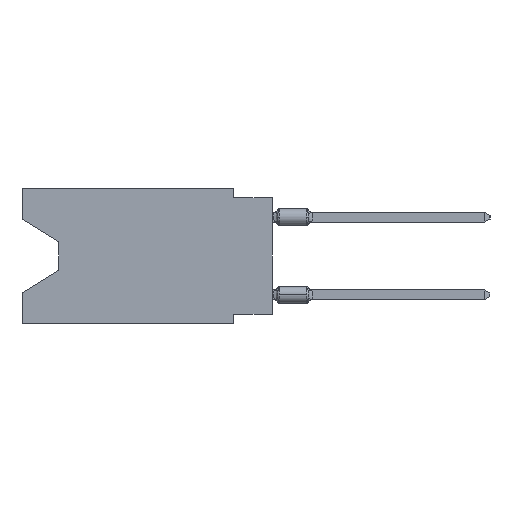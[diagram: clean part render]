
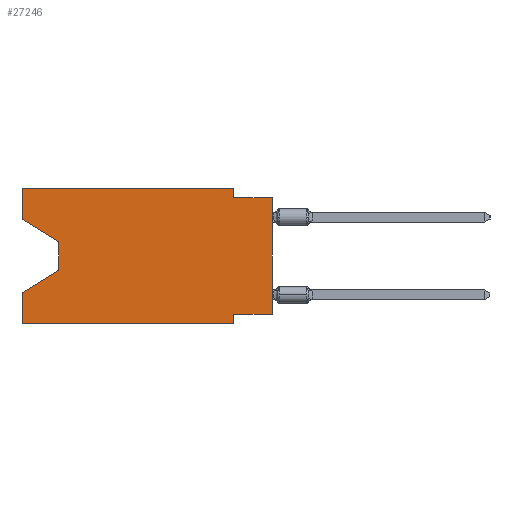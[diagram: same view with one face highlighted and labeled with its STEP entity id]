
A CAD part, left-side view. The second image highlights one B-rep face of the part: STEP entity #27246.
In plain terms, the highlighted planar face has unit normal (-1, 0, 0).
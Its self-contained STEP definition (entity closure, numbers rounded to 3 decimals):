
#243 = ORIENTED_EDGE ( 'NONE', *, *, #36101, .F. ) ;
#1244 = VERTEX_POINT ( 'NONE', #25184 ) ;
#1502 = VERTEX_POINT ( 'NONE', #13848 ) ;
#1836 = VECTOR ( 'NONE', #27882, 1000. ) ;
#2350 = PLANE ( 'NONE',  #14796 ) ;
#2396 = EDGE_CURVE ( 'NONE', #35068, #18469, #34611, .T. ) ;
#2640 = VERTEX_POINT ( 'NONE', #30639 ) ;
#2656 = CARTESIAN_POINT ( 'NONE',  ( 0., 2.54, -8.89 ) ) ;
#2669 = ORIENTED_EDGE ( 'NONE', *, *, #27727, .F. ) ;
#2722 = EDGE_CURVE ( 'NONE', #1244, #35068, #22559, .T. ) ;
#3279 = LINE ( 'NONE', #21567, #27703 ) ;
#3629 = ORIENTED_EDGE ( 'NONE', *, *, #34436, .T. ) ;
#3662 = CARTESIAN_POINT ( 'NONE',  ( 0., 16.383, 0. ) ) ;
#4240 = CARTESIAN_POINT ( 'NONE',  ( 0., 16.383, 0. ) ) ;
#4295 = VERTEX_POINT ( 'NONE', #17674 ) ;
#4804 = CARTESIAN_POINT ( 'NONE',  ( 0., 2.54, -8.89 ) ) ;
#4927 = ORIENTED_EDGE ( 'NONE', *, *, #24118, .T. ) ;
#5206 = VECTOR ( 'NONE', #33832, 1000. ) ;
#6586 = ORIENTED_EDGE ( 'NONE', *, *, #27129, .F. ) ;
#6616 = DIRECTION ( 'NONE',  ( 0., -1., 0. ) ) ;
#6967 = CARTESIAN_POINT ( 'NONE',  ( 0., 2.54, 0. ) ) ;
#7654 = CARTESIAN_POINT ( 'NONE',  ( 0., 13.97, -5.385 ) ) ;
#8058 = DIRECTION ( 'NONE',  ( 0., -1., 0. ) ) ;
#8415 = ORIENTED_EDGE ( 'NONE', *, *, #13356, .F. ) ;
#9219 = CARTESIAN_POINT ( 'NONE',  ( 0., 13.97, -5.385 ) ) ;
#9267 = EDGE_CURVE ( 'NONE', #24870, #4295, #25979, .T. ) ;
#10456 = EDGE_LOOP ( 'NONE', ( #4927, #37074, #16441, #2669, #3629, #35244, #6586, #37467, #33780, #243, #19649, #8415 ) ) ;
#11590 = DIRECTION ( 'NONE',  ( 0., 1., 0. ) ) ;
#11786 = CARTESIAN_POINT ( 'NONE',  ( 0., 16.383, 0. ) ) ;
#11973 = VECTOR ( 'NONE', #18817, 1000. ) ;
#11984 = LINE ( 'NONE', #33038, #25458 ) ;
#12676 = DIRECTION ( 'NONE',  ( 0., 0., -1. ) ) ;
#13356 = EDGE_CURVE ( 'NONE', #2640, #24870, #38759, .T. ) ;
#13848 = CARTESIAN_POINT ( 'NONE',  ( 0., 0., -8.255 ) ) ;
#13868 = DIRECTION ( 'NONE',  ( 0., -0.855, -0.519 ) ) ;
#13942 = VECTOR ( 'NONE', #14269, 1000. ) ;
#14269 = DIRECTION ( 'NONE',  ( 0., 0., -1. ) ) ;
#14352 = CARTESIAN_POINT ( 'NONE',  ( 0., 16.383, 0. ) ) ;
#14796 = AXIS2_PLACEMENT_3D ( 'NONE', #14352, #26346, #29882 ) ;
#15633 = LINE ( 'NONE', #6967, #24041 ) ;
#16441 = ORIENTED_EDGE ( 'NONE', *, *, #2396, .T. ) ;
#17026 = CARTESIAN_POINT ( 'NONE',  ( 0., 16.383, -6.852 ) ) ;
#17674 = CARTESIAN_POINT ( 'NONE',  ( 0., 2.54, 0. ) ) ;
#18214 = VECTOR ( 'NONE', #31803, 1000. ) ;
#18469 = VERTEX_POINT ( 'NONE', #17026 ) ;
#18817 = DIRECTION ( 'NONE',  ( 0., -1., 0. ) ) ;
#18866 = VECTOR ( 'NONE', #20842, 1000. ) ;
#19649 = ORIENTED_EDGE ( 'NONE', *, *, #9267, .F. ) ;
#20385 = CARTESIAN_POINT ( 'NONE',  ( 0., 0., 0. ) ) ;
#20842 = DIRECTION ( 'NONE',  ( 0., 0., 1. ) ) ;
#21118 = VECTOR ( 'NONE', #24151, 1000. ) ;
#21567 = CARTESIAN_POINT ( 'NONE',  ( 0., 0., -0.635 ) ) ;
#22088 = VERTEX_POINT ( 'NONE', #35575 ) ;
#22559 = LINE ( 'NONE', #28254, #1836 ) ;
#23543 = CARTESIAN_POINT ( 'NONE',  ( 0., 0., -0.635 ) ) ;
#23693 = EDGE_CURVE ( 'NONE', #1502, #23763, #29434, .T. ) ;
#23763 = VERTEX_POINT ( 'NONE', #23543 ) ;
#24041 = VECTOR ( 'NONE', #12676, 1000. ) ;
#24118 = EDGE_CURVE ( 'NONE', #2640, #1244, #32351, .T. ) ;
#24151 = DIRECTION ( 'NONE',  ( 0., 0., 1. ) ) ;
#24531 = LINE ( 'NONE', #3662, #21118 ) ;
#24870 = VERTEX_POINT ( 'NONE', #4240 ) ;
#25184 = CARTESIAN_POINT ( 'NONE',  ( 0., 13.97, -3.505 ) ) ;
#25458 = VECTOR ( 'NONE', #11590, 1000. ) ;
#25659 = VECTOR ( 'NONE', #13868, 1000. ) ;
#25979 = LINE ( 'NONE', #38374, #28143 ) ;
#26346 = DIRECTION ( 'NONE',  ( 1., 0., 0. ) ) ;
#26928 = FACE_OUTER_BOUND ( 'NONE', #10456, .T. ) ;
#27129 = EDGE_CURVE ( 'NONE', #1502, #30397, #11984, .T. ) ;
#27246 = ADVANCED_FACE ( 'NONE', ( #26928 ), #2350, .F. ) ;
#27703 = VECTOR ( 'NONE', #6616, 1000. ) ;
#27727 = EDGE_CURVE ( 'NONE', #29899, #18469, #24531, .T. ) ;
#27882 = DIRECTION ( 'NONE',  ( 0., 0., -1. ) ) ;
#28143 = VECTOR ( 'NONE', #8058, 1000. ) ;
#28254 = CARTESIAN_POINT ( 'NONE',  ( 0., 13.97, -3.505 ) ) ;
#29434 = LINE ( 'NONE', #20385, #18214 ) ;
#29882 = DIRECTION ( 'NONE',  ( 0., 0., -1. ) ) ;
#29899 = VERTEX_POINT ( 'NONE', #30600 ) ;
#30397 = VERTEX_POINT ( 'NONE', #37439 ) ;
#30600 = CARTESIAN_POINT ( 'NONE',  ( 0., 16.383, -8.89 ) ) ;
#30639 = CARTESIAN_POINT ( 'NONE',  ( 0., 16.383, -2.038 ) ) ;
#31013 = CARTESIAN_POINT ( 'NONE',  ( 0., 16.383, -8.89 ) ) ;
#31581 = CARTESIAN_POINT ( 'NONE',  ( 0., 16.383, -2.038 ) ) ;
#31771 = LINE ( 'NONE', #2656, #13942 ) ;
#31803 = DIRECTION ( 'NONE',  ( 0., 0., 1. ) ) ;
#32351 = LINE ( 'NONE', #31581, #25659 ) ;
#32733 = VERTEX_POINT ( 'NONE', #4804 ) ;
#33038 = CARTESIAN_POINT ( 'NONE',  ( 0., 0., -8.255 ) ) ;
#33780 = ORIENTED_EDGE ( 'NONE', *, *, #34328, .F. ) ;
#33832 = DIRECTION ( 'NONE',  ( 0., 0.855, -0.519 ) ) ;
#34328 = EDGE_CURVE ( 'NONE', #22088, #23763, #3279, .T. ) ;
#34346 = LINE ( 'NONE', #31013, #11973 ) ;
#34436 = EDGE_CURVE ( 'NONE', #29899, #32733, #34346, .T. ) ;
#34611 = LINE ( 'NONE', #7654, #5206 ) ;
#35068 = VERTEX_POINT ( 'NONE', #9219 ) ;
#35244 = ORIENTED_EDGE ( 'NONE', *, *, #35807, .F. ) ;
#35575 = CARTESIAN_POINT ( 'NONE',  ( 0., 2.54, -0.635 ) ) ;
#35807 = EDGE_CURVE ( 'NONE', #30397, #32733, #31771, .T. ) ;
#36101 = EDGE_CURVE ( 'NONE', #4295, #22088, #15633, .T. ) ;
#37074 = ORIENTED_EDGE ( 'NONE', *, *, #2722, .T. ) ;
#37439 = CARTESIAN_POINT ( 'NONE',  ( 0., 2.54, -8.255 ) ) ;
#37467 = ORIENTED_EDGE ( 'NONE', *, *, #23693, .T. ) ;
#38374 = CARTESIAN_POINT ( 'NONE',  ( 0., 16.383, 0. ) ) ;
#38759 = LINE ( 'NONE', #11786, #18866 ) ;
